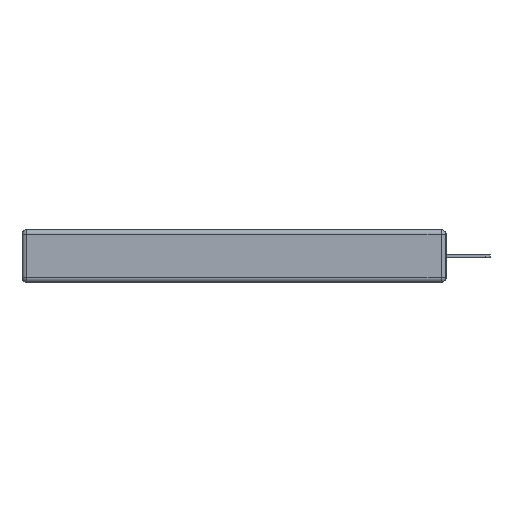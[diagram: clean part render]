
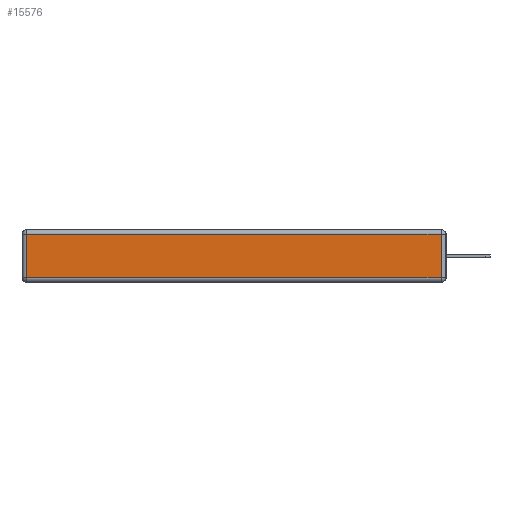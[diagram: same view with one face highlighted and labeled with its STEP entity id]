
A CAD part, left-side view. The second image highlights one B-rep face of the part: STEP entity #15576.
In plain terms, the highlighted planar face has unit normal (-1, 0, 0).
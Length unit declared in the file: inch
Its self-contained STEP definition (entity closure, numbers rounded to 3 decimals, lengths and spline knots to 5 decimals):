
#1694 = DIRECTION ( 'NONE',  ( 0., 0., 1. ) ) ;
#2139 = DIRECTION ( 'NONE',  ( 0., -1., 0. ) ) ;
#3418 = VERTEX_POINT ( 'NONE', #7031 ) ;
#4730 = ORIENTED_EDGE ( 'NONE', *, *, #12966, .T. ) ;
#4845 = VERTEX_POINT ( 'NONE', #8383 ) ;
#5099 = LINE ( 'NONE', #22484, #7668 ) ;
#5877 = ORIENTED_EDGE ( 'NONE', *, *, #26517, .T. ) ;
#6166 = DIRECTION ( 'NONE',  ( 0., 1., 0. ) ) ;
#6916 = CARTESIAN_POINT ( 'NONE',  ( 0., 0.03, -0.313 ) ) ;
#7031 = CARTESIAN_POINT ( 'NONE',  ( 0., 2.72, -0.03 ) ) ;
#7668 = VECTOR ( 'NONE', #6166, 39.37008 ) ;
#8383 = CARTESIAN_POINT ( 'NONE',  ( 0., 2.72, -0.313 ) ) ;
#9695 = DIRECTION ( 'NONE',  ( -1., 0., 0. ) ) ;
#10297 = AXIS2_PLACEMENT_3D ( 'NONE', #20138, #9695, #24163 ) ;
#10345 = CARTESIAN_POINT ( 'NONE',  ( 0., 0., -0.313 ) ) ;
#10932 = ORIENTED_EDGE ( 'NONE', *, *, #15567, .T. ) ;
#11515 = CARTESIAN_POINT ( 'NONE',  ( 0., 2.72, -0.343 ) ) ;
#12133 = VECTOR ( 'NONE', #19482, 39.37008 ) ;
#12189 = FACE_OUTER_BOUND ( 'NONE', #21324, .T. ) ;
#12598 = VERTEX_POINT ( 'NONE', #6916 ) ;
#12966 = EDGE_CURVE ( 'NONE', #3418, #4845, #19884, .T. ) ;
#13330 = LINE ( 'NONE', #10345, #24399 ) ;
#14139 = VERTEX_POINT ( 'NONE', #19644 ) ;
#15076 = LINE ( 'NONE', #22257, #17681 ) ;
#15567 = EDGE_CURVE ( 'NONE', #12598, #14139, #15076, .T. ) ;
#15576 = ADVANCED_FACE ( 'NONE', ( #12189 ), #22155, .T. ) ;
#17681 = VECTOR ( 'NONE', #1694, 39.37008 ) ;
#19482 = DIRECTION ( 'NONE',  ( 0., 0., -1. ) ) ;
#19644 = CARTESIAN_POINT ( 'NONE',  ( 0., 0.03, -0.03 ) ) ;
#19884 = LINE ( 'NONE', #11515, #12133 ) ;
#20138 = CARTESIAN_POINT ( 'NONE',  ( 0., 0., -0.343 ) ) ;
#21324 = EDGE_LOOP ( 'NONE', ( #5877, #10932, #25941, #4730 ) ) ;
#22155 = PLANE ( 'NONE',  #10297 ) ;
#22257 = CARTESIAN_POINT ( 'NONE',  ( 0., 0.03, -0.343 ) ) ;
#22484 = CARTESIAN_POINT ( 'NONE',  ( 0., 2.75, -0.03 ) ) ;
#24163 = DIRECTION ( 'NONE',  ( 0., 0., 1. ) ) ;
#24399 = VECTOR ( 'NONE', #2139, 39.37008 ) ;
#24626 = EDGE_CURVE ( 'NONE', #14139, #3418, #5099, .T. ) ;
#25941 = ORIENTED_EDGE ( 'NONE', *, *, #24626, .T. ) ;
#26517 = EDGE_CURVE ( 'NONE', #4845, #12598, #13330, .T. ) ;
